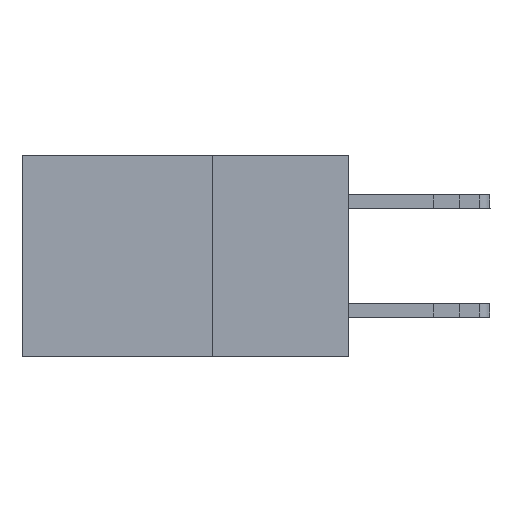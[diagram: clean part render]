
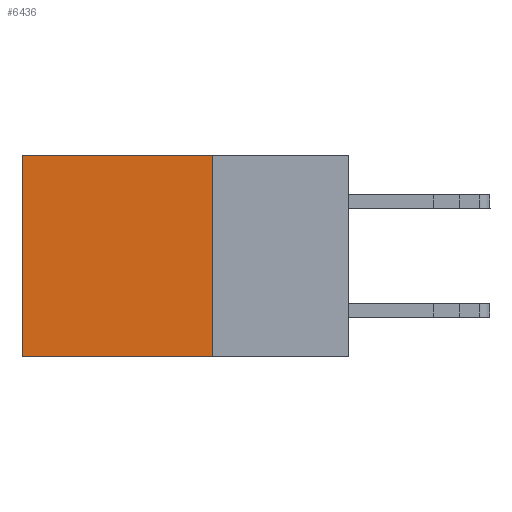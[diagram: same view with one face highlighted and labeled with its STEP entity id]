
A CAD part, left-side view. The second image highlights one B-rep face of the part: STEP entity #6436.
In plain terms, the highlighted planar face has unit normal (-1, 0, 0).
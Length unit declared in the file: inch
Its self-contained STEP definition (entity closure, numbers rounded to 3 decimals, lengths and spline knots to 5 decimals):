
#129 = VERTEX_POINT ( 'NONE', #8663 ) ;
#277 = LINE ( 'NONE', #15177, #6409 ) ;
#300 = VECTOR ( 'NONE', #3663, 39.37008 ) ;
#373 = PLANE ( 'NONE',  #2757 ) ;
#461 = FACE_OUTER_BOUND ( 'NONE', #5853, .T. ) ;
#805 = LINE ( 'NONE', #9355, #300 ) ;
#1764 = CARTESIAN_POINT ( 'NONE',  ( 0.2615, 0.25, -0.37 ) ) ;
#2296 = ORIENTED_EDGE ( 'NONE', *, *, #18215, .T. ) ;
#2578 = VERTEX_POINT ( 'NONE', #7010 ) ;
#2757 = AXIS2_PLACEMENT_3D ( 'NONE', #12035, #7854, #14815 ) ;
#2762 = VECTOR ( 'NONE', #17648, 39.37008 ) ;
#3086 = DIRECTION ( 'NONE',  ( 0., 1., 0. ) ) ;
#3663 = DIRECTION ( 'NONE',  ( 0., 0., -1. ) ) ;
#3727 = ORIENTED_EDGE ( 'NONE', *, *, #17239, .T. ) ;
#4664 = EDGE_CURVE ( 'NONE', #18239, #129, #6038, .T. ) ;
#4973 = VECTOR ( 'NONE', #3086, 39.37008 ) ;
#5113 = DIRECTION ( 'NONE',  ( 0., 1., 0. ) ) ;
#5764 = ORIENTED_EDGE ( 'NONE', *, *, #13049, .F. ) ;
#5853 = EDGE_LOOP ( 'NONE', ( #3727, #11346, #5764, #2296 ) ) ;
#6038 = LINE ( 'NONE', #1764, #4973 ) ;
#6409 = VECTOR ( 'NONE', #5113, 39.37008 ) ;
#6436 = ADVANCED_FACE ( 'NONE', ( #461 ), #373, .F. ) ;
#7010 = CARTESIAN_POINT ( 'NONE',  ( 0.2615, 0.6, 0. ) ) ;
#7854 = DIRECTION ( 'NONE',  ( 1., 0., 0. ) ) ;
#8663 = CARTESIAN_POINT ( 'NONE',  ( 0.2615, 0.6, -0.37 ) ) ;
#9236 = CARTESIAN_POINT ( 'NONE',  ( 0.2615, 0.25, 0. ) ) ;
#9355 = CARTESIAN_POINT ( 'NONE',  ( 0.2615, 0.25, -0.37 ) ) ;
#11346 = ORIENTED_EDGE ( 'NONE', *, *, #4664, .F. ) ;
#12035 = CARTESIAN_POINT ( 'NONE',  ( 0.2615, 0.25, -0.37 ) ) ;
#13049 = EDGE_CURVE ( 'NONE', #14414, #18239, #805, .T. ) ;
#14414 = VERTEX_POINT ( 'NONE', #9236 ) ;
#14815 = DIRECTION ( 'NONE',  ( 0., 0., -1. ) ) ;
#14985 = CARTESIAN_POINT ( 'NONE',  ( 0.2615, 0.6, -0.37 ) ) ;
#15177 = CARTESIAN_POINT ( 'NONE',  ( 0.2615, 0.25, 0. ) ) ;
#16227 = LINE ( 'NONE', #14985, #2762 ) ;
#17239 = EDGE_CURVE ( 'NONE', #2578, #129, #16227, .T. ) ;
#17648 = DIRECTION ( 'NONE',  ( 0., 0., -1. ) ) ;
#18122 = CARTESIAN_POINT ( 'NONE',  ( 0.2615, 0.25, -0.37 ) ) ;
#18215 = EDGE_CURVE ( 'NONE', #14414, #2578, #277, .T. ) ;
#18239 = VERTEX_POINT ( 'NONE', #18122 ) ;
